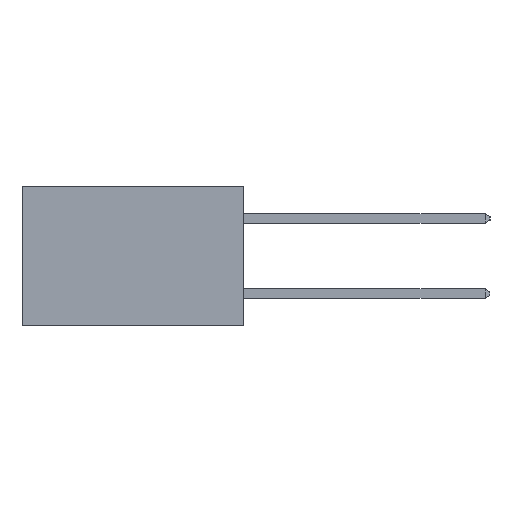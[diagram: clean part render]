
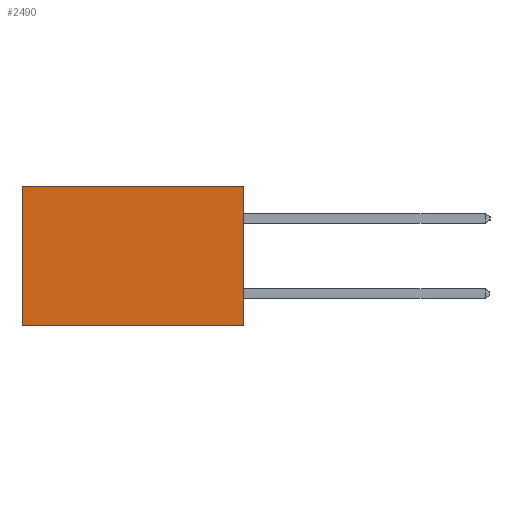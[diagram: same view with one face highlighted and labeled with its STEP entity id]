
A CAD part, left-side view. The second image highlights one B-rep face of the part: STEP entity #2490.
In plain terms, the highlighted planar face has unit normal (-1, 0, 0).
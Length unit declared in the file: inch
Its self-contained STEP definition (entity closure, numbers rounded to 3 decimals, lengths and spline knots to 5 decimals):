
#672 = EDGE_CURVE ( 'NONE', #980, #17584, #17891, .T. ) ;
#980 = VERTEX_POINT ( 'NONE', #5845 ) ;
#1159 = VERTEX_POINT ( 'NONE', #8584 ) ;
#1269 = DIRECTION ( 'NONE',  ( 0., 0., -1. ) ) ;
#1866 = VECTOR ( 'NONE', #4554, 39.37008 ) ;
#1897 = EDGE_CURVE ( 'NONE', #12644, #980, #16444, .T. ) ;
#1968 = DIRECTION ( 'NONE',  ( 1., 0., 0. ) ) ;
#2300 = DIRECTION ( 'NONE',  ( 0., 1., 0. ) ) ;
#2490 = ADVANCED_FACE ( 'NONE', ( #3202 ), #11626, .F. ) ;
#3202 = FACE_OUTER_BOUND ( 'NONE', #7273, .T. ) ;
#3275 = VECTOR ( 'NONE', #12475, 39.37008 ) ;
#3777 = DIRECTION ( 'NONE',  ( 0., 0., -1. ) ) ;
#4554 = DIRECTION ( 'NONE',  ( 0., 0., -1. ) ) ;
#5309 = EDGE_CURVE ( 'NONE', #12644, #1159, #16179, .T. ) ;
#5845 = CARTESIAN_POINT ( 'NONE',  ( 0.277, 0.59, 0. ) ) ;
#6870 = LINE ( 'NONE', #8142, #3275 ) ;
#7273 = EDGE_LOOP ( 'NONE', ( #11590, #12889, #9571, #17317 ) ) ;
#7375 = EDGE_CURVE ( 'NONE', #1159, #17584, #6870, .T. ) ;
#8142 = CARTESIAN_POINT ( 'NONE',  ( 0.277, 0., -0.37 ) ) ;
#8584 = CARTESIAN_POINT ( 'NONE',  ( 0.277, 0., -0.37 ) ) ;
#9571 = ORIENTED_EDGE ( 'NONE', *, *, #5309, .F. ) ;
#10424 = CARTESIAN_POINT ( 'NONE',  ( 0.277, 0., 0. ) ) ;
#11590 = ORIENTED_EDGE ( 'NONE', *, *, #672, .T. ) ;
#11626 = PLANE ( 'NONE',  #12439 ) ;
#12439 = AXIS2_PLACEMENT_3D ( 'NONE', #15232, #1968, #1269 ) ;
#12475 = DIRECTION ( 'NONE',  ( 0., 1., 0. ) ) ;
#12644 = VERTEX_POINT ( 'NONE', #10424 ) ;
#12889 = ORIENTED_EDGE ( 'NONE', *, *, #7375, .F. ) ;
#14383 = CARTESIAN_POINT ( 'NONE',  ( 0.277, 0.59, -0.37 ) ) ;
#15232 = CARTESIAN_POINT ( 'NONE',  ( 0.277, 0., -0.37 ) ) ;
#15875 = CARTESIAN_POINT ( 'NONE',  ( 0.277, 0., -0.37 ) ) ;
#16041 = VECTOR ( 'NONE', #2300, 39.37008 ) ;
#16179 = LINE ( 'NONE', #15875, #1866 ) ;
#16444 = LINE ( 'NONE', #16801, #16041 ) ;
#16801 = CARTESIAN_POINT ( 'NONE',  ( 0.277, 0., 0. ) ) ;
#17317 = ORIENTED_EDGE ( 'NONE', *, *, #1897, .T. ) ;
#17495 = VECTOR ( 'NONE', #3777, 39.37008 ) ;
#17584 = VERTEX_POINT ( 'NONE', #17755 ) ;
#17755 = CARTESIAN_POINT ( 'NONE',  ( 0.277, 0.59, -0.37 ) ) ;
#17891 = LINE ( 'NONE', #14383, #17495 ) ;
